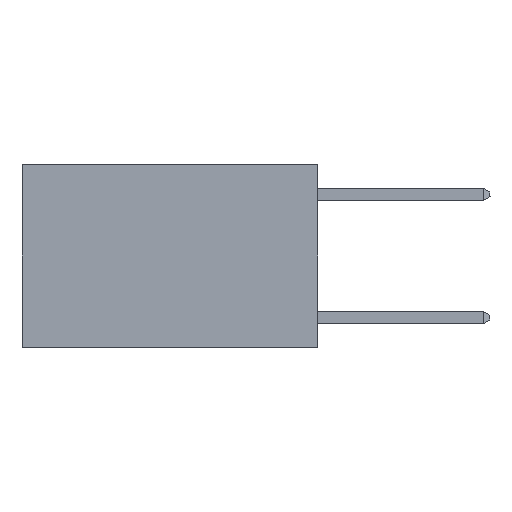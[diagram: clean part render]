
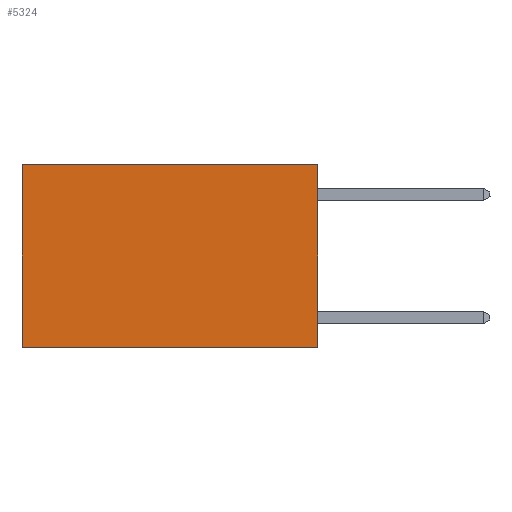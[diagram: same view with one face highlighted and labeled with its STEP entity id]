
A CAD part, left-side view. The second image highlights one B-rep face of the part: STEP entity #5324.
In plain terms, the highlighted planar face has unit normal (-1, 0, 0).
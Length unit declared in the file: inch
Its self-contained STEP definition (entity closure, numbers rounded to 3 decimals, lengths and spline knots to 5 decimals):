
#47 = ORIENTED_EDGE ( 'NONE', *, *, #4067, .T. ) ;
#118 = VECTOR ( 'NONE', #6363, 39.37008 ) ;
#339 = EDGE_CURVE ( 'NONE', #4731, #7413, #7353, .T. ) ;
#768 = AXIS2_PLACEMENT_3D ( 'NONE', #6393, #1428, #816 ) ;
#816 = DIRECTION ( 'NONE',  ( 0., 0., -1. ) ) ;
#1282 = CARTESIAN_POINT ( 'NONE',  ( 0.2625, 0.6, 0. ) ) ;
#1369 = CARTESIAN_POINT ( 'NONE',  ( 0.2625, 0.6, 0. ) ) ;
#1428 = DIRECTION ( 'NONE',  ( 1., 0., 0. ) ) ;
#1657 = LINE ( 'NONE', #2967, #3139 ) ;
#1972 = DIRECTION ( 'NONE',  ( 0., 1., 0. ) ) ;
#2093 = LINE ( 'NONE', #3190, #5739 ) ;
#2967 = CARTESIAN_POINT ( 'NONE',  ( 0.2625, 0., 0. ) ) ;
#3139 = VECTOR ( 'NONE', #6696, 39.37008 ) ;
#3190 = CARTESIAN_POINT ( 'NONE',  ( 0.2625, 0., 0. ) ) ;
#3925 = ORIENTED_EDGE ( 'NONE', *, *, #7632, .T. ) ;
#4067 = EDGE_CURVE ( 'NONE', #5128, #7413, #6333, .T. ) ;
#4265 = CARTESIAN_POINT ( 'NONE',  ( 0.2625, 0., -0.37 ) ) ;
#4539 = FACE_OUTER_BOUND ( 'NONE', #4596, .T. ) ;
#4596 = EDGE_LOOP ( 'NONE', ( #47, #5689, #4783, #3925 ) ) ;
#4731 = VERTEX_POINT ( 'NONE', #7533 ) ;
#4783 = ORIENTED_EDGE ( 'NONE', *, *, #6338, .F. ) ;
#5128 = VERTEX_POINT ( 'NONE', #1369 ) ;
#5324 = ADVANCED_FACE ( 'NONE', ( #4539 ), #6997, .F. ) ;
#5689 = ORIENTED_EDGE ( 'NONE', *, *, #339, .F. ) ;
#5739 = VECTOR ( 'NONE', #6922, 39.37008 ) ;
#6333 = LINE ( 'NONE', #1282, #118 ) ;
#6338 = EDGE_CURVE ( 'NONE', #7596, #4731, #2093, .T. ) ;
#6363 = DIRECTION ( 'NONE',  ( 0., 0., -1. ) ) ;
#6393 = CARTESIAN_POINT ( 'NONE',  ( 0.2625, 0., 0. ) ) ;
#6610 = CARTESIAN_POINT ( 'NONE',  ( 0.2625, 0., 0. ) ) ;
#6696 = DIRECTION ( 'NONE',  ( 0., 1., 0. ) ) ;
#6922 = DIRECTION ( 'NONE',  ( 0., 0., -1. ) ) ;
#6997 = PLANE ( 'NONE',  #768 ) ;
#7174 = VECTOR ( 'NONE', #1972, 39.37008 ) ;
#7353 = LINE ( 'NONE', #4265, #7174 ) ;
#7413 = VERTEX_POINT ( 'NONE', #8060 ) ;
#7533 = CARTESIAN_POINT ( 'NONE',  ( 0.2625, 0., -0.37 ) ) ;
#7596 = VERTEX_POINT ( 'NONE', #6610 ) ;
#7632 = EDGE_CURVE ( 'NONE', #7596, #5128, #1657, .T. ) ;
#8060 = CARTESIAN_POINT ( 'NONE',  ( 0.2625, 0.6, -0.37 ) ) ;
